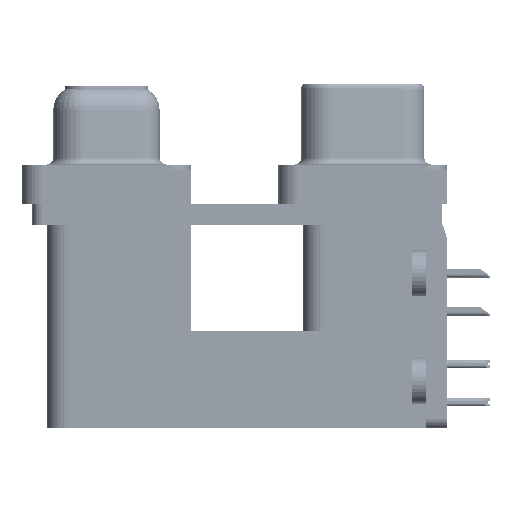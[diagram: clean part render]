
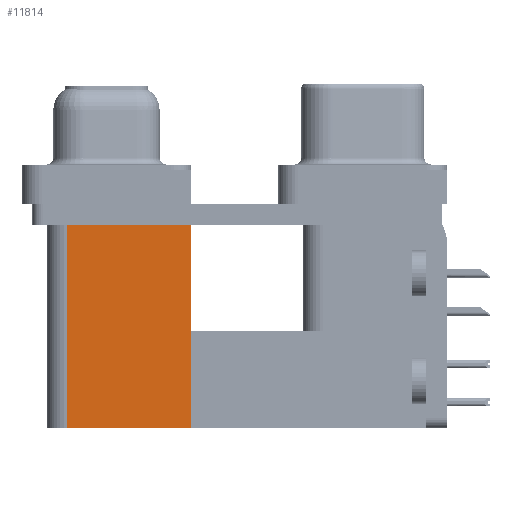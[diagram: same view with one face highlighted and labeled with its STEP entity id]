
A CAD part, left-side view. The second image highlights one B-rep face of the part: STEP entity #11814.
In plain terms, the highlighted planar face has unit normal (-1, 0, 0).
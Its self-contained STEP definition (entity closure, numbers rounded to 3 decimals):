
#1273 = FACE_OUTER_BOUND ( 'NONE', #56397, .T. ) ;
#2382 = CARTESIAN_POINT ( 'NONE',  ( 3.7, 12.775, -19.2 ) ) ;
#3054 = CARTESIAN_POINT ( 'NONE',  ( 3.7, 12.775, -19.2 ) ) ;
#5430 = CARTESIAN_POINT ( 'NONE',  ( 3.7, 12.775, -19.2 ) ) ;
#7022 = CARTESIAN_POINT ( 'NONE',  ( 3.7, 12.775, -2.5 ) ) ;
#7093 = VERTEX_POINT ( 'NONE', #47223 ) ;
#8238 = AXIS2_PLACEMENT_3D ( 'NONE', #28571, #37815, #54642 ) ;
#11814 = ADVANCED_FACE ( 'NONE', ( #1273 ), #27986, .F. ) ;
#12233 = CARTESIAN_POINT ( 'NONE',  ( 3.7, 21.975, -19.2 ) ) ;
#15088 = ORIENTED_EDGE ( 'NONE', *, *, #36888, .F. ) ;
#17958 = CARTESIAN_POINT ( 'NONE',  ( 3.7, 21.975, -19.2 ) ) ;
#18765 = LINE ( 'NONE', #23418, #47237 ) ;
#19029 = EDGE_CURVE ( 'NONE', #22680, #33068, #41929, .T. ) ;
#19518 = ORIENTED_EDGE ( 'NONE', *, *, #19029, .T. ) ;
#20914 = VERTEX_POINT ( 'NONE', #17958 ) ;
#22680 = VERTEX_POINT ( 'NONE', #2382 ) ;
#23418 = CARTESIAN_POINT ( 'NONE',  ( 3.7, 12.775, -2.5 ) ) ;
#26445 = VECTOR ( 'NONE', #53856, 1000. ) ;
#27784 = LINE ( 'NONE', #5430, #26445 ) ;
#27986 = PLANE ( 'NONE',  #8238 ) ;
#28571 = CARTESIAN_POINT ( 'NONE',  ( 3.7, 12.775, -19.2 ) ) ;
#33068 = VERTEX_POINT ( 'NONE', #7022 ) ;
#33177 = EDGE_CURVE ( 'NONE', #20914, #7093, #34305, .T. ) ;
#34305 = LINE ( 'NONE', #12233, #42035 ) ;
#36888 = EDGE_CURVE ( 'NONE', #22680, #20914, #27784, .T. ) ;
#37631 = DIRECTION ( 'NONE',  ( 0., 1., 0. ) ) ;
#37815 = DIRECTION ( 'NONE',  ( 1., 0., 0. ) ) ;
#38928 = DIRECTION ( 'NONE',  ( 0., 0., 1. ) ) ;
#41313 = ORIENTED_EDGE ( 'NONE', *, *, #44717, .T. ) ;
#41929 = LINE ( 'NONE', #3054, #42534 ) ;
#42035 = VECTOR ( 'NONE', #38928, 1000. ) ;
#42534 = VECTOR ( 'NONE', #50912, 1000. ) ;
#43251 = ORIENTED_EDGE ( 'NONE', *, *, #33177, .F. ) ;
#44717 = EDGE_CURVE ( 'NONE', #33068, #7093, #18765, .T. ) ;
#47223 = CARTESIAN_POINT ( 'NONE',  ( 3.7, 21.975, -2.5 ) ) ;
#47237 = VECTOR ( 'NONE', #37631, 1000. ) ;
#50912 = DIRECTION ( 'NONE',  ( 0., 0., 1. ) ) ;
#53856 = DIRECTION ( 'NONE',  ( 0., 1., 0. ) ) ;
#54642 = DIRECTION ( 'NONE',  ( 0., 0., -1. ) ) ;
#56397 = EDGE_LOOP ( 'NONE', ( #41313, #43251, #15088, #19518 ) ) ;
